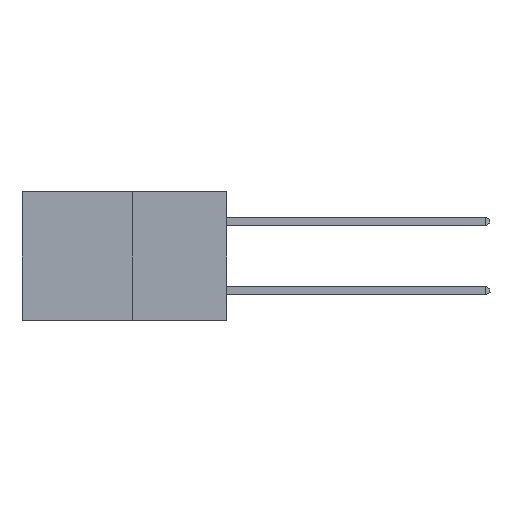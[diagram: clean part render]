
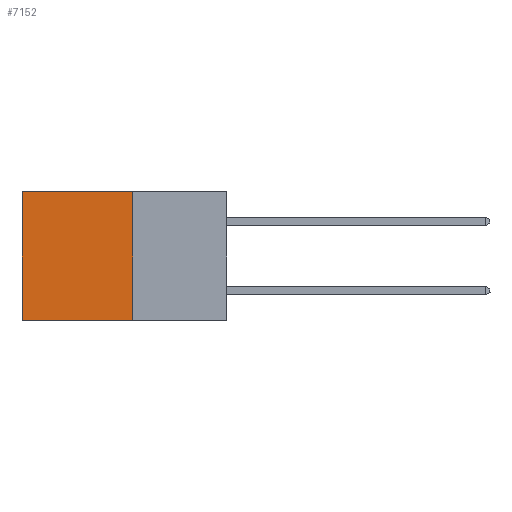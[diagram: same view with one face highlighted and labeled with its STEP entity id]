
A CAD part, left-side view. The second image highlights one B-rep face of the part: STEP entity #7152.
In plain terms, the highlighted planar face has unit normal (-1, 0, 0).
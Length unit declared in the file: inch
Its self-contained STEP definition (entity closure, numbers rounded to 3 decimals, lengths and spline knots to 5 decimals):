
#26 = CARTESIAN_POINT ( 'NONE',  ( 0.277, 0.27, -0.37 ) ) ;
#137 = LINE ( 'NONE', #1754, #6113 ) ;
#391 = VERTEX_POINT ( 'NONE', #14347 ) ;
#485 = EDGE_CURVE ( 'NONE', #9311, #391, #14517, .T. ) ;
#590 = CARTESIAN_POINT ( 'NONE',  ( 0.277, 0.59, -0.37 ) ) ;
#1073 = LINE ( 'NONE', #8788, #13587 ) ;
#1537 = DIRECTION ( 'NONE',  ( 0., 0., -1. ) ) ;
#1753 = DIRECTION ( 'NONE',  ( 0., 0., -1. ) ) ;
#1754 = CARTESIAN_POINT ( 'NONE',  ( 0.277, 0.27, -0.37 ) ) ;
#2006 = EDGE_LOOP ( 'NONE', ( #5496, #5467, #11540, #11686 ) ) ;
#2881 = DIRECTION ( 'NONE',  ( 0., 1., 0. ) ) ;
#2995 = VERTEX_POINT ( 'NONE', #26 ) ;
#5154 = DIRECTION ( 'NONE',  ( 1., 0., 0. ) ) ;
#5373 = LINE ( 'NONE', #590, #8640 ) ;
#5467 = ORIENTED_EDGE ( 'NONE', *, *, #13422, .F. ) ;
#5496 = ORIENTED_EDGE ( 'NONE', *, *, #11431, .T. ) ;
#5694 = VERTEX_POINT ( 'NONE', #7159 ) ;
#6113 = VECTOR ( 'NONE', #6531, 39.37008 ) ;
#6531 = DIRECTION ( 'NONE',  ( 0., 1., 0. ) ) ;
#7152 = ADVANCED_FACE ( 'NONE', ( #12803 ), #12444, .F. ) ;
#7159 = CARTESIAN_POINT ( 'NONE',  ( 0.277, 0.59, -0.37 ) ) ;
#7655 = VECTOR ( 'NONE', #2881, 39.37008 ) ;
#8037 = CARTESIAN_POINT ( 'NONE',  ( 0.277, 0.27, -0.37 ) ) ;
#8640 = VECTOR ( 'NONE', #1753, 39.37008 ) ;
#8788 = CARTESIAN_POINT ( 'NONE',  ( 0.277, 0.27, -0.37 ) ) ;
#9311 = VERTEX_POINT ( 'NONE', #9731 ) ;
#9416 = CARTESIAN_POINT ( 'NONE',  ( 0.277, 0.27, 0. ) ) ;
#9682 = DIRECTION ( 'NONE',  ( 0., 0., -1. ) ) ;
#9731 = CARTESIAN_POINT ( 'NONE',  ( 0.277, 0.27, 0. ) ) ;
#11431 = EDGE_CURVE ( 'NONE', #391, #5694, #5373, .T. ) ;
#11540 = ORIENTED_EDGE ( 'NONE', *, *, #11976, .F. ) ;
#11686 = ORIENTED_EDGE ( 'NONE', *, *, #485, .T. ) ;
#11976 = EDGE_CURVE ( 'NONE', #9311, #2995, #1073, .T. ) ;
#12155 = AXIS2_PLACEMENT_3D ( 'NONE', #8037, #5154, #9682 ) ;
#12444 = PLANE ( 'NONE',  #12155 ) ;
#12803 = FACE_OUTER_BOUND ( 'NONE', #2006, .T. ) ;
#13422 = EDGE_CURVE ( 'NONE', #2995, #5694, #137, .T. ) ;
#13587 = VECTOR ( 'NONE', #1537, 39.37008 ) ;
#14347 = CARTESIAN_POINT ( 'NONE',  ( 0.277, 0.59, 0. ) ) ;
#14517 = LINE ( 'NONE', #9416, #7655 ) ;
